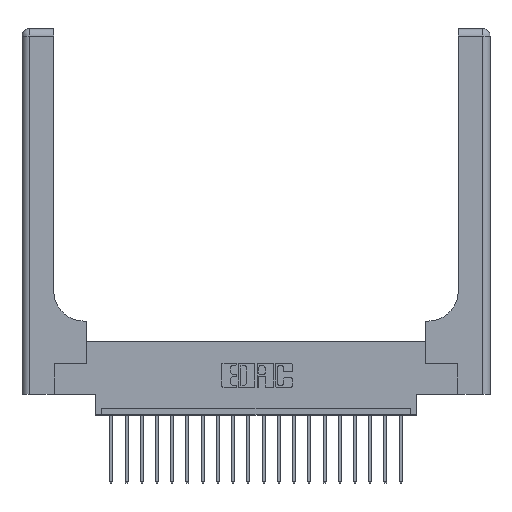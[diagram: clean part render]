
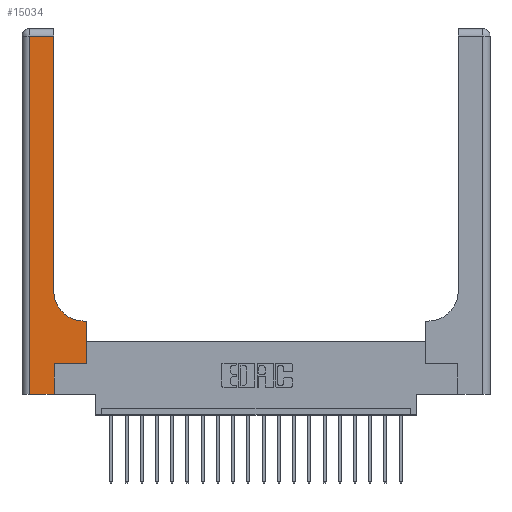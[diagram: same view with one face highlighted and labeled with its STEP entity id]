
A CAD part, top view. The second image highlights one B-rep face of the part: STEP entity #15034.
In plain terms, the highlighted planar face has unit normal (0, 0, 1).
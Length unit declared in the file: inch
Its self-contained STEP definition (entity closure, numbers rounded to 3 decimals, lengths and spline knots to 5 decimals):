
#536 = AXIS2_PLACEMENT_3D ( 'NONE', #9025, #17343, #7637 ) ;
#787 = PLANE ( 'NONE',  #536 ) ;
#1206 = ORIENTED_EDGE ( 'NONE', *, *, #18226, .T. ) ;
#1408 = DIRECTION ( 'NONE',  ( 0., 1., 0. ) ) ;
#1475 = VERTEX_POINT ( 'NONE', #20077 ) ;
#1504 = EDGE_CURVE ( 'NONE', #9334, #8627, #4277, .T. ) ;
#1733 = CARTESIAN_POINT ( 'NONE',  ( 0., 2.94, 0.37 ) ) ;
#1962 = VECTOR ( 'NONE', #19316, 39.37008 ) ;
#2673 = CARTESIAN_POINT ( 'NONE',  ( 0.51, 0.85, 0.37 ) ) ;
#2800 = EDGE_CURVE ( 'NONE', #8627, #7153, #17111, .T. ) ;
#3268 = DIRECTION ( 'NONE',  ( 1., 0., 0. ) ) ;
#3302 = CARTESIAN_POINT ( 'NONE',  ( 0.26, 2.94, 0.37 ) ) ;
#3534 = CARTESIAN_POINT ( 'NONE',  ( 0.26, 0.85, 0.37 ) ) ;
#4138 = EDGE_CURVE ( 'NONE', #1475, #9334, #19405, .T. ) ;
#4259 = ORIENTED_EDGE ( 'NONE', *, *, #4138, .T. ) ;
#4277 = LINE ( 'NONE', #4688, #1962 ) ;
#4688 = CARTESIAN_POINT ( 'NONE',  ( 0.265, 0., 0.37 ) ) ;
#5148 = EDGE_CURVE ( 'NONE', #17894, #11637, #12235, .T. ) ;
#5580 = DIRECTION ( 'NONE',  ( 1., 0., 0. ) ) ;
#5783 = AXIS2_PLACEMENT_3D ( 'NONE', #2673, #16873, #5580 ) ;
#5791 = VECTOR ( 'NONE', #9462, 39.37008 ) ;
#6051 = CARTESIAN_POINT ( 'NONE',  ( 0.26, 0.6, 0.37 ) ) ;
#6099 = EDGE_CURVE ( 'NONE', #11637, #15728, #11435, .T. ) ;
#6345 = CARTESIAN_POINT ( 'NONE',  ( 0.26, 3., 0.37 ) ) ;
#6913 = ORIENTED_EDGE ( 'NONE', *, *, #16545, .T. ) ;
#7153 = VERTEX_POINT ( 'NONE', #14797 ) ;
#7304 = DIRECTION ( 'NONE',  ( 1., 0., 0. ) ) ;
#7637 = DIRECTION ( 'NONE',  ( -1., 0., 0. ) ) ;
#7715 = CARTESIAN_POINT ( 'NONE',  ( 0.265, 0.25, 0.37 ) ) ;
#7791 = VERTEX_POINT ( 'NONE', #20565 ) ;
#8627 = VERTEX_POINT ( 'NONE', #21005 ) ;
#8842 = CARTESIAN_POINT ( 'NONE',  ( 0.06, 2.94, 0.37 ) ) ;
#9025 = CARTESIAN_POINT ( 'NONE',  ( 0., 3., 0.37 ) ) ;
#9334 = VERTEX_POINT ( 'NONE', #18701 ) ;
#9462 = DIRECTION ( 'NONE',  ( -1., 0., 0. ) ) ;
#9764 = LINE ( 'NONE', #21081, #18635 ) ;
#10495 = DIRECTION ( 'NONE',  ( 0., -1., 0. ) ) ;
#10812 = LINE ( 'NONE', #17322, #21108 ) ;
#11435 = LINE ( 'NONE', #6345, #18579 ) ;
#11453 = ORIENTED_EDGE ( 'NONE', *, *, #6099, .T. ) ;
#11637 = VERTEX_POINT ( 'NONE', #3534 ) ;
#11671 = FACE_OUTER_BOUND ( 'NONE', #18182, .T. ) ;
#12235 = CIRCLE ( 'NONE', #5783, 0.25 ) ;
#12307 = VERTEX_POINT ( 'NONE', #8842 ) ;
#12836 = DIRECTION ( 'NONE',  ( -1., 0., 0. ) ) ;
#12867 = VECTOR ( 'NONE', #3268, 39.37008 ) ;
#13095 = VECTOR ( 'NONE', #7304, 39.37008 ) ;
#13730 = ORIENTED_EDGE ( 'NONE', *, *, #5148, .T. ) ;
#14340 = LINE ( 'NONE', #1733, #17982 ) ;
#14544 = DIRECTION ( 'NONE',  ( 0., 1., 0. ) ) ;
#14695 = CARTESIAN_POINT ( 'NONE',  ( 0., 0., 0.37 ) ) ;
#14797 = CARTESIAN_POINT ( 'NONE',  ( 0.528, 0.25, 0.37 ) ) ;
#15034 = ADVANCED_FACE ( 'NONE', ( #11671 ), #787, .F. ) ;
#15205 = EDGE_CURVE ( 'NONE', #7153, #7791, #9764, .T. ) ;
#15671 = ORIENTED_EDGE ( 'NONE', *, *, #2800, .T. ) ;
#15724 = ORIENTED_EDGE ( 'NONE', *, *, #15205, .T. ) ;
#15728 = VERTEX_POINT ( 'NONE', #3302 ) ;
#16189 = CARTESIAN_POINT ( 'NONE',  ( 0.51, 0.6, 0.37 ) ) ;
#16382 = ORIENTED_EDGE ( 'NONE', *, *, #1504, .T. ) ;
#16528 = ORIENTED_EDGE ( 'NONE', *, *, #20262, .T. ) ;
#16545 = EDGE_CURVE ( 'NONE', #15728, #12307, #14340, .T. ) ;
#16873 = DIRECTION ( 'NONE',  ( 0., 0., -1. ) ) ;
#17111 = LINE ( 'NONE', #7715, #13095 ) ;
#17322 = CARTESIAN_POINT ( 'NONE',  ( 0.06, 3., 0.37 ) ) ;
#17343 = DIRECTION ( 'NONE',  ( 0., 0., -1. ) ) ;
#17894 = VERTEX_POINT ( 'NONE', #16189 ) ;
#17982 = VECTOR ( 'NONE', #12836, 39.37008 ) ;
#18182 = EDGE_LOOP ( 'NONE', ( #11453, #6913, #16528, #4259, #16382, #15671, #15724, #1206, #13730 ) ) ;
#18226 = EDGE_CURVE ( 'NONE', #7791, #17894, #19274, .T. ) ;
#18579 = VECTOR ( 'NONE', #1408, 39.37008 ) ;
#18635 = VECTOR ( 'NONE', #14544, 39.37008 ) ;
#18701 = CARTESIAN_POINT ( 'NONE',  ( 0.265, 0., 0.37 ) ) ;
#19274 = LINE ( 'NONE', #6051, #5791 ) ;
#19316 = DIRECTION ( 'NONE',  ( 0., 1., 0. ) ) ;
#19405 = LINE ( 'NONE', #14695, #12867 ) ;
#20077 = CARTESIAN_POINT ( 'NONE',  ( 0.06, 0., 0.37 ) ) ;
#20262 = EDGE_CURVE ( 'NONE', #12307, #1475, #10812, .T. ) ;
#20565 = CARTESIAN_POINT ( 'NONE',  ( 0.528, 0.6, 0.37 ) ) ;
#21005 = CARTESIAN_POINT ( 'NONE',  ( 0.265, 0.25, 0.37 ) ) ;
#21081 = CARTESIAN_POINT ( 'NONE',  ( 0.528, 0.25, 0.37 ) ) ;
#21108 = VECTOR ( 'NONE', #10495, 39.37008 ) ;
